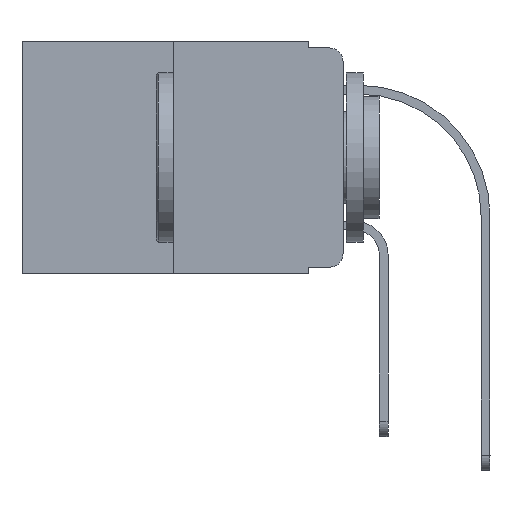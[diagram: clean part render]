
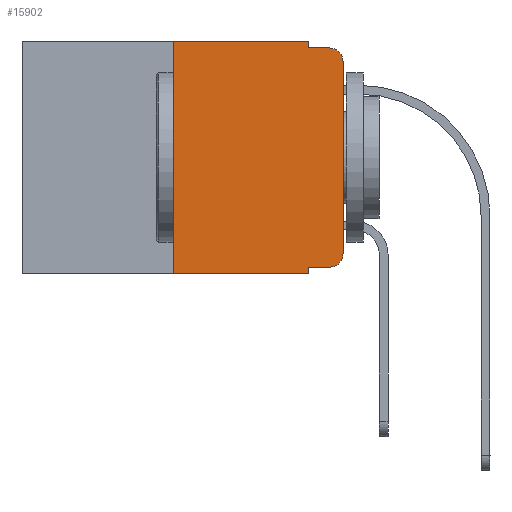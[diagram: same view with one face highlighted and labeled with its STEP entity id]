
A CAD part, left-side view. The second image highlights one B-rep face of the part: STEP entity #15902.
In plain terms, the highlighted planar face has unit normal (-1, 0, 0).
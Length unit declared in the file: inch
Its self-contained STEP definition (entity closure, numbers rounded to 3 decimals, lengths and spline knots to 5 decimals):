
#16 = ORIENTED_EDGE ( 'NONE', *, *, #16208, .F. ) ;
#21 = DIRECTION ( 'NONE',  ( 0., 0., -1. ) ) ;
#451 = VECTOR ( 'NONE', #10578, 39.37008 ) ;
#464 = ORIENTED_EDGE ( 'NONE', *, *, #13635, .F. ) ;
#485 = EDGE_CURVE ( 'NONE', #743, #6332, #9042, .T. ) ;
#513 = EDGE_CURVE ( 'NONE', #11640, #6577, #11830, .T. ) ;
#743 = VERTEX_POINT ( 'NONE', #11278 ) ;
#1471 = VERTEX_POINT ( 'NONE', #17581 ) ;
#1647 = VECTOR ( 'NONE', #7716, 39.37008 ) ;
#1676 = EDGE_LOOP ( 'NONE', ( #11386, #10617, #16336, #7094, #464, #16, #11638, #14535, #4984, #6751 ) ) ;
#1800 = CARTESIAN_POINT ( 'NONE',  ( 0., 0.02, -0.333 ) ) ;
#1811 = CARTESIAN_POINT ( 'NONE',  ( 0., 0.25, 0. ) ) ;
#2142 = AXIS2_PLACEMENT_3D ( 'NONE', #5640, #3059, #6803 ) ;
#2528 = DIRECTION ( 'NONE',  ( 1., 0., 0. ) ) ;
#3059 = DIRECTION ( 'NONE',  ( -1., 0., 0. ) ) ;
#3235 = LINE ( 'NONE', #1811, #11558 ) ;
#3535 = DIRECTION ( 'NONE',  ( 0., 0., -1. ) ) ;
#4738 = EDGE_CURVE ( 'NONE', #1471, #12698, #17288, .T. ) ;
#4863 = EDGE_CURVE ( 'NONE', #11314, #11640, #12270, .T. ) ;
#4984 = ORIENTED_EDGE ( 'NONE', *, *, #485, .T. ) ;
#5010 = CARTESIAN_POINT ( 'NONE',  ( 0., 0.02, -0.01 ) ) ;
#5024 = VECTOR ( 'NONE', #21, 39.37008 ) ;
#5451 = EDGE_CURVE ( 'NONE', #12698, #6577, #10268, .T. ) ;
#5640 = CARTESIAN_POINT ( 'NONE',  ( 0., 0.02, -0.313 ) ) ;
#5911 = DIRECTION ( 'NONE',  ( 0., 0., 1. ) ) ;
#6235 = VERTEX_POINT ( 'NONE', #13609 ) ;
#6304 = DIRECTION ( 'NONE',  ( 0., 0., -1. ) ) ;
#6332 = VERTEX_POINT ( 'NONE', #1800 ) ;
#6410 = AXIS2_PLACEMENT_3D ( 'NONE', #15872, #2528, #6304 ) ;
#6525 = DIRECTION ( 'NONE',  ( 0., -1., 0. ) ) ;
#6577 = VERTEX_POINT ( 'NONE', #5010 ) ;
#6658 = CARTESIAN_POINT ( 'NONE',  ( 0., 0.051, 0. ) ) ;
#6751 = ORIENTED_EDGE ( 'NONE', *, *, #7571, .T. ) ;
#6803 = DIRECTION ( 'NONE',  ( 0., 0., -1. ) ) ;
#6864 = VECTOR ( 'NONE', #15643, 39.37008 ) ;
#6891 = CARTESIAN_POINT ( 'NONE',  ( 0., 0.051, 0. ) ) ;
#7094 = ORIENTED_EDGE ( 'NONE', *, *, #4863, .F. ) ;
#7571 = EDGE_CURVE ( 'NONE', #6332, #1471, #17562, .T. ) ;
#7716 = DIRECTION ( 'NONE',  ( 0., 0., 1. ) ) ;
#8293 = CARTESIAN_POINT ( 'NONE',  ( 0., 0.051, 0. ) ) ;
#8553 = AXIS2_PLACEMENT_3D ( 'NONE', #14453, #16881, #3535 ) ;
#8699 = VERTEX_POINT ( 'NONE', #13557 ) ;
#8760 = CARTESIAN_POINT ( 'NONE',  ( 0., 0.473, 0. ) ) ;
#9042 = LINE ( 'NONE', #10392, #12148 ) ;
#9249 = PLANE ( 'NONE',  #6410 ) ;
#9307 = CARTESIAN_POINT ( 'NONE',  ( 0., 0.051, -0.01 ) ) ;
#9473 = CARTESIAN_POINT ( 'NONE',  ( 0., 0., -0.03 ) ) ;
#10037 = LINE ( 'NONE', #8760, #6864 ) ;
#10076 = LINE ( 'NONE', #15516, #17533 ) ;
#10268 = CIRCLE ( 'NONE', #8553, 0.02 ) ;
#10392 = CARTESIAN_POINT ( 'NONE',  ( 0., 0.051, -0.333 ) ) ;
#10578 = DIRECTION ( 'NONE',  ( 0., -1., 0. ) ) ;
#10617 = ORIENTED_EDGE ( 'NONE', *, *, #5451, .T. ) ;
#11154 = DIRECTION ( 'NONE',  ( 0., 0., -1. ) ) ;
#11278 = CARTESIAN_POINT ( 'NONE',  ( 0., 0.051, -0.333 ) ) ;
#11314 = VERTEX_POINT ( 'NONE', #8293 ) ;
#11386 = ORIENTED_EDGE ( 'NONE', *, *, #4738, .T. ) ;
#11558 = VECTOR ( 'NONE', #5911, 39.37008 ) ;
#11638 = ORIENTED_EDGE ( 'NONE', *, *, #15741, .T. ) ;
#11640 = VERTEX_POINT ( 'NONE', #11870 ) ;
#11667 = CARTESIAN_POINT ( 'NONE',  ( 0., 0.25, 0. ) ) ;
#11830 = LINE ( 'NONE', #9307, #451 ) ;
#11870 = CARTESIAN_POINT ( 'NONE',  ( 0., 0.051, -0.01 ) ) ;
#12148 = VECTOR ( 'NONE', #6525, 39.37008 ) ;
#12270 = LINE ( 'NONE', #6891, #5024 ) ;
#12308 = LINE ( 'NONE', #6658, #16902 ) ;
#12698 = VERTEX_POINT ( 'NONE', #9473 ) ;
#13358 = FACE_OUTER_BOUND ( 'NONE', #1676, .T. ) ;
#13557 = CARTESIAN_POINT ( 'NONE',  ( 0., 0.051, -0.343 ) ) ;
#13609 = CARTESIAN_POINT ( 'NONE',  ( 0., 0.25, -0.343 ) ) ;
#13635 = EDGE_CURVE ( 'NONE', #17260, #11314, #10037, .T. ) ;
#14323 = EDGE_CURVE ( 'NONE', #743, #8699, #12308, .T. ) ;
#14453 = CARTESIAN_POINT ( 'NONE',  ( 0., 0.02, -0.03 ) ) ;
#14511 = CARTESIAN_POINT ( 'NONE',  ( 0., 0., 0. ) ) ;
#14535 = ORIENTED_EDGE ( 'NONE', *, *, #14323, .F. ) ;
#15516 = CARTESIAN_POINT ( 'NONE',  ( 0., 0.473, -0.343 ) ) ;
#15643 = DIRECTION ( 'NONE',  ( 0., -1., 0. ) ) ;
#15741 = EDGE_CURVE ( 'NONE', #6235, #8699, #10076, .T. ) ;
#15872 = CARTESIAN_POINT ( 'NONE',  ( 0., 0.473, 0. ) ) ;
#15902 = ADVANCED_FACE ( 'NONE', ( #13358 ), #9249, .F. ) ;
#16208 = EDGE_CURVE ( 'NONE', #6235, #17260, #3235, .T. ) ;
#16336 = ORIENTED_EDGE ( 'NONE', *, *, #513, .F. ) ;
#16881 = DIRECTION ( 'NONE',  ( -1., 0., 0. ) ) ;
#16902 = VECTOR ( 'NONE', #11154, 39.37008 ) ;
#17037 = DIRECTION ( 'NONE',  ( 0., -1., 0. ) ) ;
#17260 = VERTEX_POINT ( 'NONE', #11667 ) ;
#17288 = LINE ( 'NONE', #14511, #1647 ) ;
#17533 = VECTOR ( 'NONE', #17037, 39.37008 ) ;
#17562 = CIRCLE ( 'NONE', #2142, 0.02 ) ;
#17581 = CARTESIAN_POINT ( 'NONE',  ( 0., 0., -0.313 ) ) ;
